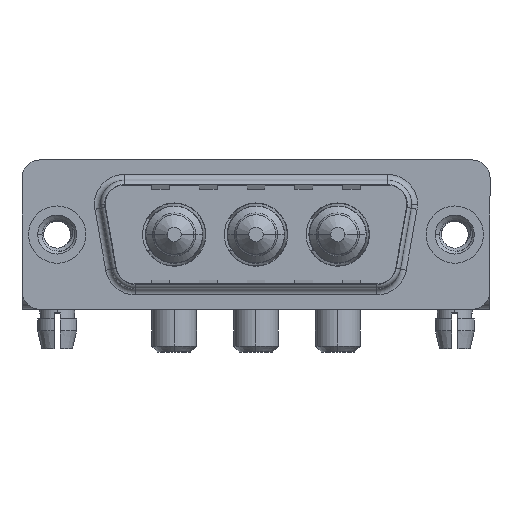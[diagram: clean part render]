
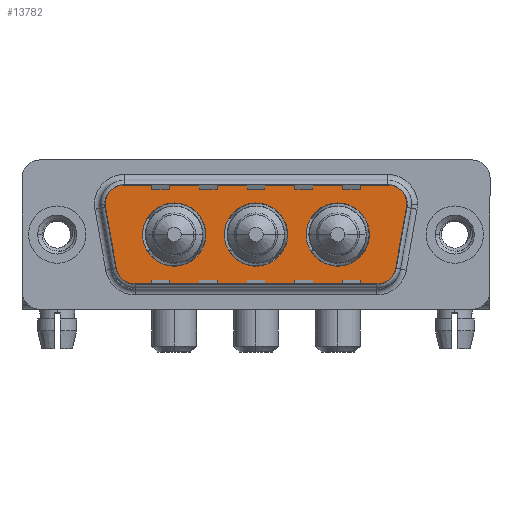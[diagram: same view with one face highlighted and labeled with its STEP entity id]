
A CAD part, top view. The second image highlights one B-rep face of the part: STEP entity #13782.
In plain terms, the highlighted planar face has unit normal (0, 0, 1).
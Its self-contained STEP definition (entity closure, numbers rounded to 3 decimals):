
#158 = ORIENTED_EDGE ( 'NONE', *, *, #6426, .T. ) ;
#328 = DIRECTION ( 'NONE',  ( 0., 0., 1. ) ) ;
#334 = VERTEX_POINT ( 'NONE', #9761 ) ;
#372 = EDGE_CURVE ( 'NONE', #11915, #2782, #9259, .T. ) ;
#493 = DIRECTION ( 'NONE',  ( 0., 0., 1. ) ) ;
#583 = DIRECTION ( 'NONE',  ( 0.174, -0.985, 0. ) ) ;
#631 = DIRECTION ( 'NONE',  ( -1., 0., 0. ) ) ;
#673 = CARTESIAN_POINT ( 'NONE',  ( 7.15, 0., 0. ) ) ;
#698 = VERTEX_POINT ( 'NONE', #8195 ) ;
#938 = VERTEX_POINT ( 'NONE', #10280 ) ;
#1044 = VERTEX_POINT ( 'NONE', #11656 ) ;
#1196 = ORIENTED_EDGE ( 'NONE', *, *, #372, .F. ) ;
#1285 = EDGE_LOOP ( 'NONE', ( #13950, #158, #8254, #8183, #4182, #12382, #11527, #7850, #8936 ) ) ;
#1307 = EDGE_CURVE ( 'NONE', #2782, #11915, #4806, .T. ) ;
#1323 = CIRCLE ( 'NONE', #5287, 2.65 ) ;
#1485 = DIRECTION ( 'NONE',  ( 0., 0., 1. ) ) ;
#1553 = VERTEX_POINT ( 'NONE', #12863 ) ;
#1726 = ORIENTED_EDGE ( 'NONE', *, *, #2500, .F. ) ;
#2056 = LINE ( 'NONE', #15106, #7021 ) ;
#2067 = DIRECTION ( 'NONE',  ( 1., 0., 0. ) ) ;
#2316 = LINE ( 'NONE', #14286, #3142 ) ;
#2500 = EDGE_CURVE ( 'NONE', #7105, #15078, #5096, .T. ) ;
#2757 = FACE_BOUND ( 'NONE', #9623, .T. ) ;
#2782 = VERTEX_POINT ( 'NONE', #10990 ) ;
#2832 = CARTESIAN_POINT ( 'NONE',  ( 26.866, -2.9, 0. ) ) ;
#2851 = DIRECTION ( 'NONE',  ( 0.174, 0.985, 0. ) ) ;
#2918 = PLANE ( 'NONE',  #7255 ) ;
#3078 = DIRECTION ( 'NONE',  ( 0., 0., 1. ) ) ;
#3079 = CIRCLE ( 'NONE', #7504, 2. ) ;
#3142 = VECTOR ( 'NONE', #10899, 1000. ) ;
#3262 = FACE_BOUND ( 'NONE', #8923, .T. ) ;
#3314 = AXIS2_PLACEMENT_3D ( 'NONE', #9826, #1485, #7507 ) ;
#3484 = EDGE_CURVE ( 'NONE', #938, #4698, #2316, .T. ) ;
#3542 = CARTESIAN_POINT ( 'NONE',  ( 28.836, -3.247, 0. ) ) ;
#3564 = CIRCLE ( 'NONE', #3314, 2. ) ;
#3729 = ORIENTED_EDGE ( 'NONE', *, *, #14624, .F. ) ;
#3918 = DIRECTION ( 'NONE',  ( 1., 0., 0. ) ) ;
#4182 = ORIENTED_EDGE ( 'NONE', *, *, #3484, .T. ) ;
#4291 = CARTESIAN_POINT ( 'NONE',  ( 26.15, 0., 0. ) ) ;
#4482 = EDGE_CURVE ( 'NONE', #1044, #698, #13995, .T. ) ;
#4698 = VERTEX_POINT ( 'NONE', #8978 ) ;
#4806 = CIRCLE ( 'NONE', #9739, 2.65 ) ;
#4820 = DIRECTION ( 'NONE',  ( -1., 0., 0. ) ) ;
#4922 = ORIENTED_EDGE ( 'NONE', *, *, #12378, .F. ) ;
#5095 = DIRECTION ( 'NONE',  ( 0., 0., 1. ) ) ;
#5096 = CIRCLE ( 'NONE', #11267, 2.65 ) ;
#5185 = AXIS2_PLACEMENT_3D ( 'NONE', #11078, #493, #13536 ) ;
#5287 = AXIS2_PLACEMENT_3D ( 'NONE', #11421, #10189, #2067 ) ;
#5399 = CARTESIAN_POINT ( 'NONE',  ( 16.65, 0., 0. ) ) ;
#5781 = AXIS2_PLACEMENT_3D ( 'NONE', #8717, #3078, #13500 ) ;
#6316 = DIRECTION ( 'NONE',  ( 1., 0., 0. ) ) ;
#6358 = DIRECTION ( 'NONE',  ( 0., 0., 1. ) ) ;
#6426 = EDGE_CURVE ( 'NONE', #14377, #7389, #7639, .T. ) ;
#6567 = DIRECTION ( 'NONE',  ( 0., 0., 1. ) ) ;
#7021 = VECTOR ( 'NONE', #8163, 1000. ) ;
#7105 = VERTEX_POINT ( 'NONE', #12990 ) ;
#7255 = AXIS2_PLACEMENT_3D ( 'NONE', #2832, #10295, #10937 ) ;
#7349 = CARTESIAN_POINT ( 'NONE',  ( 26.866, -4.9, 0. ) ) ;
#7358 = EDGE_CURVE ( 'NONE', #4698, #7820, #10847, .T. ) ;
#7389 = VERTEX_POINT ( 'NONE', #12234 ) ;
#7504 = AXIS2_PLACEMENT_3D ( 'NONE', #9974, #6567, #631 ) ;
#7507 = DIRECTION ( 'NONE',  ( -1., 0., 0. ) ) ;
#7612 = AXIS2_PLACEMENT_3D ( 'NONE', #14467, #328, #4820 ) ;
#7639 = LINE ( 'NONE', #7712, #7896 ) ;
#7712 = CARTESIAN_POINT ( 'NONE',  ( 29.859, 2.553, 0. ) ) ;
#7820 = VERTEX_POINT ( 'NONE', #14747 ) ;
#7850 = ORIENTED_EDGE ( 'NONE', *, *, #4482, .T. ) ;
#7896 = VECTOR ( 'NONE', #2851, 1000. ) ;
#8163 = DIRECTION ( 'NONE',  ( 1., 0., 0. ) ) ;
#8183 = ORIENTED_EDGE ( 'NONE', *, *, #10499, .T. ) ;
#8195 = CARTESIAN_POINT ( 'NONE',  ( 6.434, -4.9, 0. ) ) ;
#8254 = ORIENTED_EDGE ( 'NONE', *, *, #12755, .T. ) ;
#8386 = DIRECTION ( 'NONE',  ( 0., 0., 1. ) ) ;
#8546 = CARTESIAN_POINT ( 'NONE',  ( 9.8, 0., 0. ) ) ;
#8700 = FACE_BOUND ( 'NONE', #15055, .T. ) ;
#8717 = CARTESIAN_POINT ( 'NONE',  ( 26.866, -2.9, 0. ) ) ;
#8753 = CIRCLE ( 'NONE', #14681, 2.65 ) ;
#8853 = CARTESIAN_POINT ( 'NONE',  ( 3.441, 2.553, 0. ) ) ;
#8923 = EDGE_LOOP ( 'NONE', ( #1726, #13250 ) ) ;
#8936 = ORIENTED_EDGE ( 'NONE', *, *, #14717, .T. ) ;
#8978 = CARTESIAN_POINT ( 'NONE',  ( 5.411, 4.9, 0. ) ) ;
#9063 = VERTEX_POINT ( 'NONE', #7349 ) ;
#9259 = CIRCLE ( 'NONE', #15169, 2.65 ) ;
#9623 = EDGE_LOOP ( 'NONE', ( #1196, #10920 ) ) ;
#9739 = AXIS2_PLACEMENT_3D ( 'NONE', #13422, #5095, #12116 ) ;
#9761 = CARTESIAN_POINT ( 'NONE',  ( 19.3, 0., 0. ) ) ;
#9826 = CARTESIAN_POINT ( 'NONE',  ( 27.889, 2.9, 0. ) ) ;
#9974 = CARTESIAN_POINT ( 'NONE',  ( 27.889, 2.9, 0. ) ) ;
#10005 = AXIS2_PLACEMENT_3D ( 'NONE', #8546, #8386, #3918 ) ;
#10189 = DIRECTION ( 'NONE',  ( 0., 0., 1. ) ) ;
#10280 = CARTESIAN_POINT ( 'NONE',  ( 27.889, 4.9, 0. ) ) ;
#10295 = DIRECTION ( 'NONE',  ( 0., 0., 1. ) ) ;
#10478 = CIRCLE ( 'NONE', #5781, 2. ) ;
#10499 = EDGE_CURVE ( 'NONE', #1553, #938, #3564, .T. ) ;
#10847 = CIRCLE ( 'NONE', #5185, 2. ) ;
#10899 = DIRECTION ( 'NONE',  ( -1., 0., 0. ) ) ;
#10920 = ORIENTED_EDGE ( 'NONE', *, *, #1307, .F. ) ;
#10937 = DIRECTION ( 'NONE',  ( 1., 0., 0. ) ) ;
#10990 = CARTESIAN_POINT ( 'NONE',  ( 20.85, 0., 0. ) ) ;
#11002 = CARTESIAN_POINT ( 'NONE',  ( 23.5, 0., 0. ) ) ;
#11078 = CARTESIAN_POINT ( 'NONE',  ( 5.411, 2.9, 0. ) ) ;
#11172 = LINE ( 'NONE', #8853, #14879 ) ;
#11178 = VERTEX_POINT ( 'NONE', #12944 ) ;
#11237 = DIRECTION ( 'NONE',  ( 1., 0., 0. ) ) ;
#11267 = AXIS2_PLACEMENT_3D ( 'NONE', #15152, #11539, #12834 ) ;
#11421 = CARTESIAN_POINT ( 'NONE',  ( 16.65, 0., 0. ) ) ;
#11527 = ORIENTED_EDGE ( 'NONE', *, *, #11873, .T. ) ;
#11539 = DIRECTION ( 'NONE',  ( 0., 0., 1. ) ) ;
#11656 = CARTESIAN_POINT ( 'NONE',  ( 4.464, -3.247, 0. ) ) ;
#11873 = EDGE_CURVE ( 'NONE', #7820, #1044, #11172, .T. ) ;
#11915 = VERTEX_POINT ( 'NONE', #4291 ) ;
#12116 = DIRECTION ( 'NONE',  ( 1., 0., 0. ) ) ;
#12234 = CARTESIAN_POINT ( 'NONE',  ( 29.859, 2.553, 0. ) ) ;
#12378 = EDGE_CURVE ( 'NONE', #334, #11178, #1323, .T. ) ;
#12382 = ORIENTED_EDGE ( 'NONE', *, *, #7358, .T. ) ;
#12755 = EDGE_CURVE ( 'NONE', #7389, #1553, #3079, .T. ) ;
#12834 = DIRECTION ( 'NONE',  ( 1., 0., 0. ) ) ;
#12863 = CARTESIAN_POINT ( 'NONE',  ( 29.889, 2.9, 0. ) ) ;
#12944 = CARTESIAN_POINT ( 'NONE',  ( 14., 0., 0. ) ) ;
#12990 = CARTESIAN_POINT ( 'NONE',  ( 12.45, 0., 0. ) ) ;
#13190 = EDGE_CURVE ( 'NONE', #9063, #14377, #10478, .T. ) ;
#13192 = CIRCLE ( 'NONE', #10005, 2.65 ) ;
#13250 = ORIENTED_EDGE ( 'NONE', *, *, #14876, .F. ) ;
#13422 = CARTESIAN_POINT ( 'NONE',  ( 23.5, 0., 0. ) ) ;
#13481 = FACE_OUTER_BOUND ( 'NONE', #1285, .T. ) ;
#13500 = DIRECTION ( 'NONE',  ( 1., 0., 0. ) ) ;
#13536 = DIRECTION ( 'NONE',  ( 1., 0., 0. ) ) ;
#13642 = DIRECTION ( 'NONE',  ( 0., 0., 1. ) ) ;
#13782 = ADVANCED_FACE ( 'NONE', ( #8700, #2757, #3262, #13481 ), #2918, .T. ) ;
#13950 = ORIENTED_EDGE ( 'NONE', *, *, #13190, .T. ) ;
#13995 = CIRCLE ( 'NONE', #7612, 2. ) ;
#14286 = CARTESIAN_POINT ( 'NONE',  ( 5.411, 4.9, 0. ) ) ;
#14377 = VERTEX_POINT ( 'NONE', #3542 ) ;
#14467 = CARTESIAN_POINT ( 'NONE',  ( 6.434, -2.9, 0. ) ) ;
#14624 = EDGE_CURVE ( 'NONE', #11178, #334, #8753, .T. ) ;
#14681 = AXIS2_PLACEMENT_3D ( 'NONE', #5399, #13642, #6316 ) ;
#14717 = EDGE_CURVE ( 'NONE', #698, #9063, #2056, .T. ) ;
#14747 = CARTESIAN_POINT ( 'NONE',  ( 3.441, 2.553, 0. ) ) ;
#14876 = EDGE_CURVE ( 'NONE', #15078, #7105, #13192, .T. ) ;
#14879 = VECTOR ( 'NONE', #583, 1000. ) ;
#15055 = EDGE_LOOP ( 'NONE', ( #4922, #3729 ) ) ;
#15078 = VERTEX_POINT ( 'NONE', #673 ) ;
#15106 = CARTESIAN_POINT ( 'NONE',  ( 6.434, -4.9, 0. ) ) ;
#15152 = CARTESIAN_POINT ( 'NONE',  ( 9.8, 0., 0. ) ) ;
#15169 = AXIS2_PLACEMENT_3D ( 'NONE', #11002, #6358, #11237 ) ;
